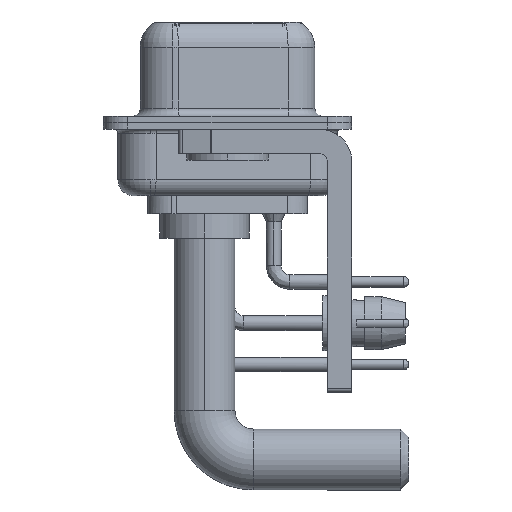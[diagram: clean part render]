
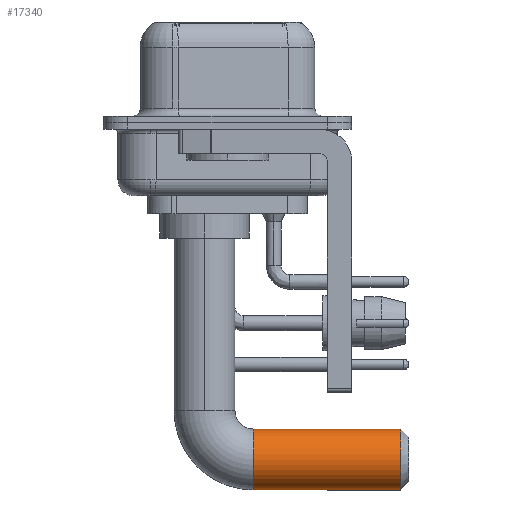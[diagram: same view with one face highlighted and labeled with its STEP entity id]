
A CAD part, left-side view. The second image highlights one B-rep face of the part: STEP entity #17340.
In plain terms, the highlighted cylindrical face has radius 1.875 mm (diameter 3.75 mm), a partial arc.
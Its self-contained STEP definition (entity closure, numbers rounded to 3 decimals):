
#2311 = CARTESIAN_POINT ( 'NONE',  ( 0., -12.07, -11.755 ) ) ;
#5073 = AXIS2_PLACEMENT_3D ( 'NONE', #16849, #28112, #17541 ) ;
#5760 = VERTEX_POINT ( 'NONE', #29222 ) ;
#6007 = DIRECTION ( 'NONE',  ( -1., 0., 0. ) ) ;
#7268 = CIRCLE ( 'NONE', #30434, 1.875 ) ;
#9658 = ORIENTED_EDGE ( 'NONE', *, *, #24066, .T. ) ;
#9803 = CIRCLE ( 'NONE', #10365, 1.875 ) ;
#9994 = CARTESIAN_POINT ( 'NONE',  ( 0., -12.07, -13.63 ) ) ;
#10365 = AXIS2_PLACEMENT_3D ( 'NONE', #9994, #15500, #34187 ) ;
#10496 = CARTESIAN_POINT ( 'NONE',  ( 0., -12.07, -15.505 ) ) ;
#11538 = FACE_OUTER_BOUND ( 'NONE', #22773, .T. ) ;
#12054 = CYLINDRICAL_SURFACE ( 'NONE', #5073, 1.875 ) ;
#12164 = EDGE_CURVE ( 'NONE', #29115, #31541, #20478, .T. ) ;
#12757 = VECTOR ( 'NONE', #17830, 1000. ) ;
#14961 = LINE ( 'NONE', #23062, #21559 ) ;
#15500 = DIRECTION ( 'NONE',  ( 0., 1., 0. ) ) ;
#16849 = CARTESIAN_POINT ( 'NONE',  ( 0., -3., -13.63 ) ) ;
#17340 = ADVANCED_FACE ( 'NONE', ( #11538 ), #12054, .T. ) ;
#17541 = DIRECTION ( 'NONE',  ( 0., 0., -1. ) ) ;
#17830 = DIRECTION ( 'NONE',  ( 0., -1., 0. ) ) ;
#18979 = VERTEX_POINT ( 'NONE', #10496 ) ;
#19475 = CARTESIAN_POINT ( 'NONE',  ( 0., -3., -13.63 ) ) ;
#20439 = DIRECTION ( 'NONE',  ( 0., -1., 0. ) ) ;
#20478 = LINE ( 'NONE', #31221, #12757 ) ;
#21559 = VECTOR ( 'NONE', #20439, 1000. ) ;
#22694 = ORIENTED_EDGE ( 'NONE', *, *, #29258, .T. ) ;
#22773 = EDGE_LOOP ( 'NONE', ( #32467, #9658, #26742, #22694 ) ) ;
#23062 = CARTESIAN_POINT ( 'NONE',  ( 0., -3., -15.505 ) ) ;
#24066 = EDGE_CURVE ( 'NONE', #29115, #5760, #7268, .T. ) ;
#26387 = EDGE_CURVE ( 'NONE', #5760, #18979, #14961, .T. ) ;
#26742 = ORIENTED_EDGE ( 'NONE', *, *, #26387, .T. ) ;
#27856 = CARTESIAN_POINT ( 'NONE',  ( 0., -3., -11.755 ) ) ;
#28112 = DIRECTION ( 'NONE',  ( 0., -1., 0. ) ) ;
#29115 = VERTEX_POINT ( 'NONE', #27856 ) ;
#29222 = CARTESIAN_POINT ( 'NONE',  ( 0., -3., -15.505 ) ) ;
#29258 = EDGE_CURVE ( 'NONE', #18979, #31541, #9803, .T. ) ;
#30230 = DIRECTION ( 'NONE',  ( 0., -1., 0. ) ) ;
#30434 = AXIS2_PLACEMENT_3D ( 'NONE', #19475, #30230, #6007 ) ;
#31221 = CARTESIAN_POINT ( 'NONE',  ( 0., -3., -11.755 ) ) ;
#31541 = VERTEX_POINT ( 'NONE', #2311 ) ;
#32467 = ORIENTED_EDGE ( 'NONE', *, *, #12164, .F. ) ;
#34187 = DIRECTION ( 'NONE',  ( 0., 0., -1. ) ) ;
